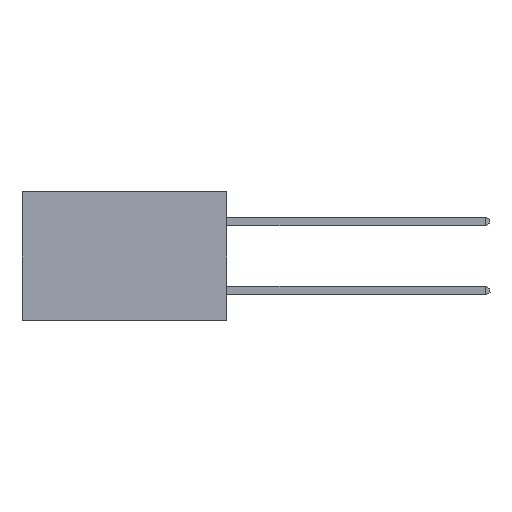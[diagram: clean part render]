
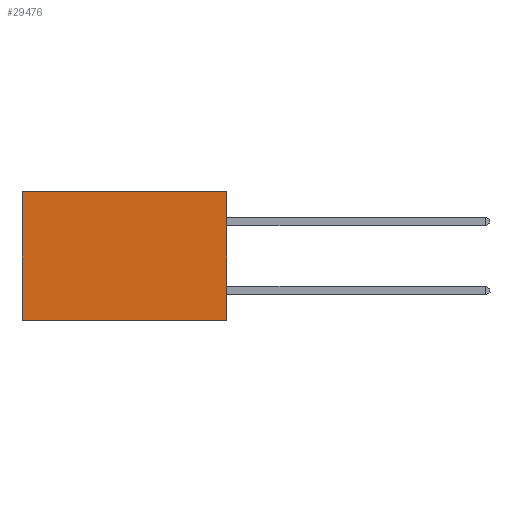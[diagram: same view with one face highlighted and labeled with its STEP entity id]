
A CAD part, left-side view. The second image highlights one B-rep face of the part: STEP entity #29476.
In plain terms, the highlighted planar face has unit normal (-1, 0, 0).
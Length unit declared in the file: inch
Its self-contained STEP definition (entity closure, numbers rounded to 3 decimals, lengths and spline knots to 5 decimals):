
#1372 = CARTESIAN_POINT ( 'NONE',  ( 0.277, 0., -0.37 ) ) ;
#2089 = CARTESIAN_POINT ( 'NONE',  ( 0.277, 0.59, -0.37 ) ) ;
#3588 = LINE ( 'NONE', #23361, #22059 ) ;
#3726 = FACE_OUTER_BOUND ( 'NONE', #6132, .T. ) ;
#3941 = DIRECTION ( 'NONE',  ( 0., 0., -1. ) ) ;
#4730 = VERTEX_POINT ( 'NONE', #32445 ) ;
#4829 = VERTEX_POINT ( 'NONE', #29821 ) ;
#5421 = ORIENTED_EDGE ( 'NONE', *, *, #17089, .F. ) ;
#6132 = EDGE_LOOP ( 'NONE', ( #26157, #5421, #7750, #24637 ) ) ;
#6807 = LINE ( 'NONE', #2089, #12369 ) ;
#7365 = CARTESIAN_POINT ( 'NONE',  ( 0.277, 0., -0.37 ) ) ;
#7750 = ORIENTED_EDGE ( 'NONE', *, *, #11989, .F. ) ;
#8348 = CARTESIAN_POINT ( 'NONE',  ( 0.277, 0., 0. ) ) ;
#9901 = DIRECTION ( 'NONE',  ( 0., 0., -1. ) ) ;
#11196 = EDGE_CURVE ( 'NONE', #11233, #19471, #31750, .T. ) ;
#11233 = VERTEX_POINT ( 'NONE', #31029 ) ;
#11989 = EDGE_CURVE ( 'NONE', #11233, #4730, #22226, .T. ) ;
#12369 = VECTOR ( 'NONE', #27161, 39.37008 ) ;
#12891 = CARTESIAN_POINT ( 'NONE',  ( 0.277, 0.59, 0. ) ) ;
#17089 = EDGE_CURVE ( 'NONE', #4730, #4829, #3588, .T. ) ;
#17337 = PLANE ( 'NONE',  #25089 ) ;
#19471 = VERTEX_POINT ( 'NONE', #12891 ) ;
#22059 = VECTOR ( 'NONE', #25885, 39.37008 ) ;
#22226 = LINE ( 'NONE', #1372, #28152 ) ;
#23361 = CARTESIAN_POINT ( 'NONE',  ( 0.277, 0., -0.37 ) ) ;
#24637 = ORIENTED_EDGE ( 'NONE', *, *, #11196, .T. ) ;
#24848 = DIRECTION ( 'NONE',  ( 1., 0., 0. ) ) ;
#25089 = AXIS2_PLACEMENT_3D ( 'NONE', #7365, #24848, #9901 ) ;
#25298 = EDGE_CURVE ( 'NONE', #19471, #4829, #6807, .T. ) ;
#25790 = VECTOR ( 'NONE', #25807, 39.37008 ) ;
#25807 = DIRECTION ( 'NONE',  ( 0., 1., 0. ) ) ;
#25885 = DIRECTION ( 'NONE',  ( 0., 1., 0. ) ) ;
#26157 = ORIENTED_EDGE ( 'NONE', *, *, #25298, .T. ) ;
#27161 = DIRECTION ( 'NONE',  ( 0., 0., -1. ) ) ;
#28152 = VECTOR ( 'NONE', #3941, 39.37008 ) ;
#29476 = ADVANCED_FACE ( 'NONE', ( #3726 ), #17337, .F. ) ;
#29821 = CARTESIAN_POINT ( 'NONE',  ( 0.277, 0.59, -0.37 ) ) ;
#31029 = CARTESIAN_POINT ( 'NONE',  ( 0.277, 0., 0. ) ) ;
#31750 = LINE ( 'NONE', #8348, #25790 ) ;
#32445 = CARTESIAN_POINT ( 'NONE',  ( 0.277, 0., -0.37 ) ) ;
